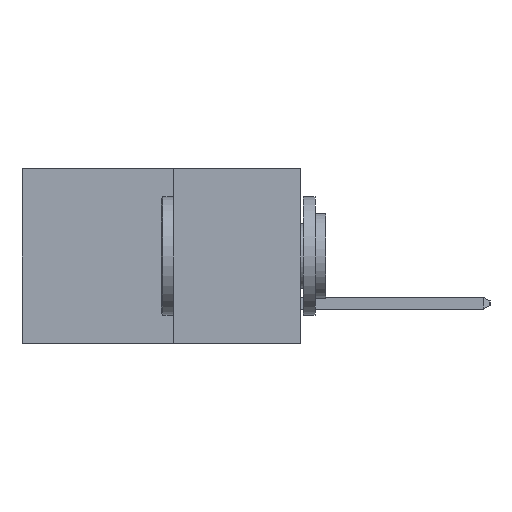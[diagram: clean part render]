
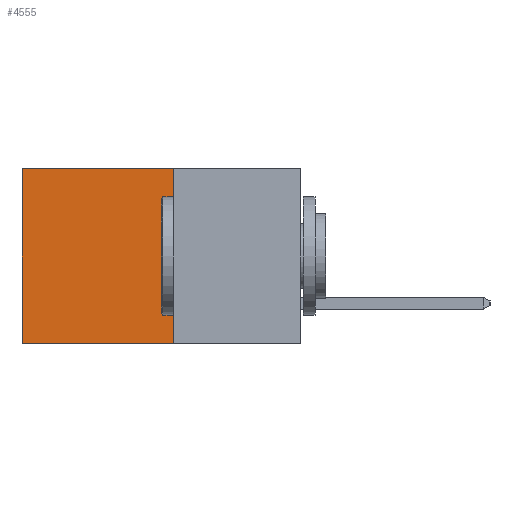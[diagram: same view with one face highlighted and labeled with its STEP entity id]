
A CAD part, left-side view. The second image highlights one B-rep face of the part: STEP entity #4555.
In plain terms, the highlighted planar face has unit normal (-1, 0, 0).
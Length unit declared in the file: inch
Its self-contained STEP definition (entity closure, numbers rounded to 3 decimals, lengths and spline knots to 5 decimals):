
#123 = EDGE_CURVE ( 'NONE', #11050, #7538, #14452, .T. ) ;
#1344 = ORIENTED_EDGE ( 'NONE', *, *, #14490, .T. ) ;
#1431 = ORIENTED_EDGE ( 'NONE', *, *, #123, .F. ) ;
#1473 = ORIENTED_EDGE ( 'NONE', *, *, #12213, .F. ) ;
#1478 = ORIENTED_EDGE ( 'NONE', *, *, #3612, .T. ) ;
#1835 = EDGE_LOOP ( 'NONE', ( #1344, #1431, #1473, #1478 ) ) ;
#2318 = LINE ( 'NONE', #9509, #8631 ) ;
#2561 = CARTESIAN_POINT ( 'NONE',  ( 0.277, 0.27, -0.37 ) ) ;
#2711 = PLANE ( 'NONE',  #11461 ) ;
#3612 = EDGE_CURVE ( 'NONE', #12392, #10010, #2318, .T. ) ;
#4555 = ADVANCED_FACE ( 'NONE', ( #15427 ), #2711, .F. ) ;
#4912 = DIRECTION ( 'NONE',  ( 0., 1., 0. ) ) ;
#5048 = CARTESIAN_POINT ( 'NONE',  ( 0.277, 0.27, 0. ) ) ;
#5952 = LINE ( 'NONE', #6681, #15341 ) ;
#6681 = CARTESIAN_POINT ( 'NONE',  ( 0.277, 0.59, -0.37 ) ) ;
#7241 = DIRECTION ( 'NONE',  ( 0., 0., -1. ) ) ;
#7538 = VERTEX_POINT ( 'NONE', #8755 ) ;
#7962 = DIRECTION ( 'NONE',  ( 0., 0., -1. ) ) ;
#8162 = CARTESIAN_POINT ( 'NONE',  ( 0.277, 0.27, -0.37 ) ) ;
#8625 = CARTESIAN_POINT ( 'NONE',  ( 0.277, 0.59, 0. ) ) ;
#8631 = VECTOR ( 'NONE', #11319, 39.37008 ) ;
#8755 = CARTESIAN_POINT ( 'NONE',  ( 0.277, 0.59, -0.37 ) ) ;
#9509 = CARTESIAN_POINT ( 'NONE',  ( 0.277, 0.27, 0. ) ) ;
#9689 = CARTESIAN_POINT ( 'NONE',  ( 0.277, 0.27, -0.37 ) ) ;
#10010 = VERTEX_POINT ( 'NONE', #8625 ) ;
#11050 = VERTEX_POINT ( 'NONE', #8162 ) ;
#11282 = VECTOR ( 'NONE', #4912, 39.37008 ) ;
#11319 = DIRECTION ( 'NONE',  ( 0., 1., 0. ) ) ;
#11461 = AXIS2_PLACEMENT_3D ( 'NONE', #2561, #14237, #7241 ) ;
#12213 = EDGE_CURVE ( 'NONE', #12392, #11050, #15564, .T. ) ;
#12392 = VERTEX_POINT ( 'NONE', #5048 ) ;
#14237 = DIRECTION ( 'NONE',  ( 1., 0., 0. ) ) ;
#14326 = CARTESIAN_POINT ( 'NONE',  ( 0.277, 0.27, -0.37 ) ) ;
#14452 = LINE ( 'NONE', #14326, #11282 ) ;
#14490 = EDGE_CURVE ( 'NONE', #10010, #7538, #5952, .T. ) ;
#14503 = DIRECTION ( 'NONE',  ( 0., 0., -1. ) ) ;
#15185 = VECTOR ( 'NONE', #14503, 39.37008 ) ;
#15341 = VECTOR ( 'NONE', #7962, 39.37008 ) ;
#15427 = FACE_OUTER_BOUND ( 'NONE', #1835, .T. ) ;
#15564 = LINE ( 'NONE', #9689, #15185 ) ;
